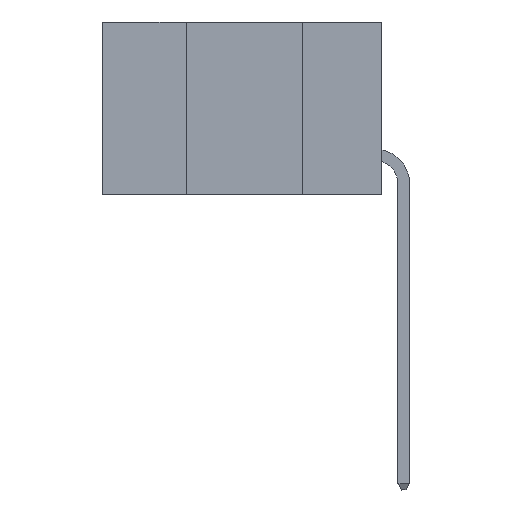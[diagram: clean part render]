
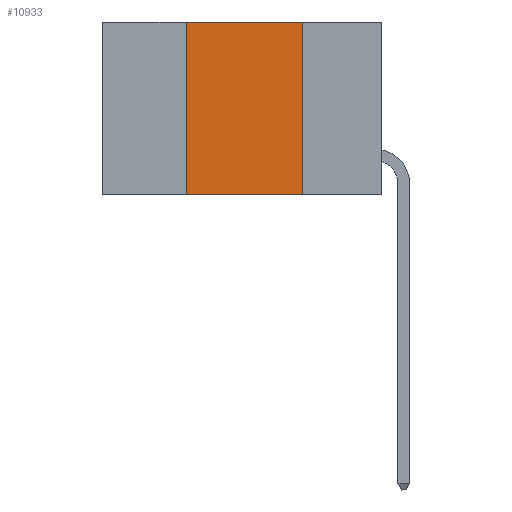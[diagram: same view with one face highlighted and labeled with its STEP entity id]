
A CAD part, left-side view. The second image highlights one B-rep face of the part: STEP entity #10933.
In plain terms, the highlighted planar face has unit normal (-1, 0, 0).
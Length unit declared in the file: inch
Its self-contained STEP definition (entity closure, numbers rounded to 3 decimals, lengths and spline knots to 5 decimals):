
#3 = VERTEX_POINT ( 'NONE', #25128 ) ;
#111 = CARTESIAN_POINT ( 'NONE',  ( 0., 0.6, 0. ) ) ;
#1772 = CARTESIAN_POINT ( 'NONE',  ( 0., 0.17, -0.37 ) ) ;
#1974 = VECTOR ( 'NONE', #5528, 39.37008 ) ;
#4201 = LINE ( 'NONE', #41668, #11533 ) ;
#5528 = DIRECTION ( 'NONE',  ( 0., -1., 0. ) ) ;
#6487 = CARTESIAN_POINT ( 'NONE',  ( 0., 0.42, 0. ) ) ;
#7733 = VERTEX_POINT ( 'NONE', #1772 ) ;
#8082 = ORIENTED_EDGE ( 'NONE', *, *, #23220, .F. ) ;
#10933 = ADVANCED_FACE ( 'NONE', ( #37814 ), #27881, .F. ) ;
#11533 = VECTOR ( 'NONE', #13915, 39.37008 ) ;
#12053 = EDGE_LOOP ( 'NONE', ( #34569, #8082, #17756, #41056 ) ) ;
#12100 = EDGE_CURVE ( 'NONE', #28410, #3, #12366, .T. ) ;
#12366 = LINE ( 'NONE', #6487, #30572 ) ;
#12853 = EDGE_CURVE ( 'NONE', #43530, #7733, #22877, .T. ) ;
#13915 = DIRECTION ( 'NONE',  ( 0., -1., 0. ) ) ;
#15056 = CARTESIAN_POINT ( 'NONE',  ( 0., 0.17, 0. ) ) ;
#16332 = DIRECTION ( 'NONE',  ( 0., 0., -1. ) ) ;
#17756 = ORIENTED_EDGE ( 'NONE', *, *, #12100, .F. ) ;
#19706 = CARTESIAN_POINT ( 'NONE',  ( 0., 0.17, 0. ) ) ;
#22451 = CARTESIAN_POINT ( 'NONE',  ( 0., 0.6, -0.37 ) ) ;
#22877 = LINE ( 'NONE', #19706, #38545 ) ;
#23220 = EDGE_CURVE ( 'NONE', #3, #43530, #4201, .T. ) ;
#23990 = AXIS2_PLACEMENT_3D ( 'NONE', #111, #30374, #34880 ) ;
#25128 = CARTESIAN_POINT ( 'NONE',  ( 0., 0.42, 0. ) ) ;
#27881 = PLANE ( 'NONE',  #23990 ) ;
#28410 = VERTEX_POINT ( 'NONE', #37550 ) ;
#29738 = DIRECTION ( 'NONE',  ( 0., 0., 1. ) ) ;
#30374 = DIRECTION ( 'NONE',  ( 1., 0., 0. ) ) ;
#30572 = VECTOR ( 'NONE', #29738, 39.37008 ) ;
#32176 = LINE ( 'NONE', #22451, #1974 ) ;
#34569 = ORIENTED_EDGE ( 'NONE', *, *, #12853, .F. ) ;
#34722 = EDGE_CURVE ( 'NONE', #28410, #7733, #32176, .T. ) ;
#34880 = DIRECTION ( 'NONE',  ( 0., 0., -1. ) ) ;
#37550 = CARTESIAN_POINT ( 'NONE',  ( 0., 0.42, -0.37 ) ) ;
#37814 = FACE_OUTER_BOUND ( 'NONE', #12053, .T. ) ;
#38545 = VECTOR ( 'NONE', #16332, 39.37008 ) ;
#41056 = ORIENTED_EDGE ( 'NONE', *, *, #34722, .T. ) ;
#41668 = CARTESIAN_POINT ( 'NONE',  ( 0., 0.6, 0. ) ) ;
#43530 = VERTEX_POINT ( 'NONE', #15056 ) ;
